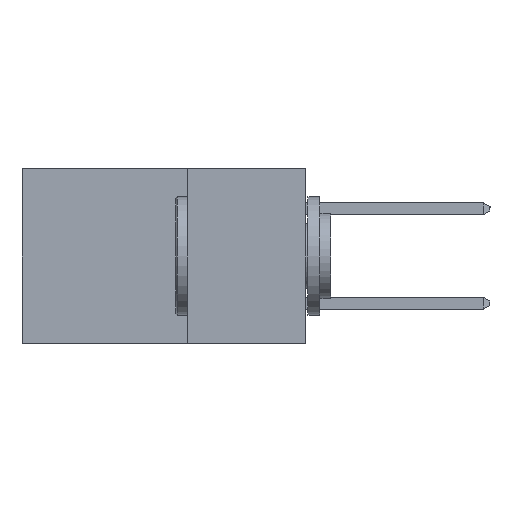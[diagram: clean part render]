
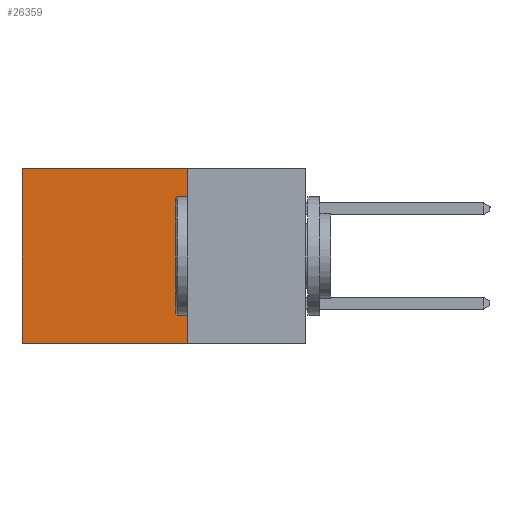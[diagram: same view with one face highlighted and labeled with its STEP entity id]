
A CAD part, left-side view. The second image highlights one B-rep face of the part: STEP entity #26359.
In plain terms, the highlighted planar face has unit normal (-1, 0, 0).
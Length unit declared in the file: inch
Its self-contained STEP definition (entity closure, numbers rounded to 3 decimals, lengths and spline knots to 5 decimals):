
#502 = CARTESIAN_POINT ( 'NONE',  ( 0.2615, 0.25, -0.37 ) ) ;
#1599 = EDGE_CURVE ( 'NONE', #26156, #15115, #1630, .T. ) ;
#1630 = LINE ( 'NONE', #23669, #22161 ) ;
#2135 = LINE ( 'NONE', #6465, #19818 ) ;
#2148 = LINE ( 'NONE', #24849, #10229 ) ;
#2182 = ORIENTED_EDGE ( 'NONE', *, *, #1599, .F. ) ;
#2357 = LINE ( 'NONE', #16408, #9030 ) ;
#4839 = PLANE ( 'NONE',  #10345 ) ;
#6465 = CARTESIAN_POINT ( 'NONE',  ( 0.2615, 0.6, -0.37 ) ) ;
#7989 = EDGE_CURVE ( 'NONE', #15115, #23376, #2148, .T. ) ;
#9030 = VECTOR ( 'NONE', #10595, 39.37008 ) ;
#9242 = VERTEX_POINT ( 'NONE', #22430 ) ;
#10229 = VECTOR ( 'NONE', #14302, 39.37008 ) ;
#10345 = AXIS2_PLACEMENT_3D ( 'NONE', #14966, #15353, #21310 ) ;
#10379 = CARTESIAN_POINT ( 'NONE',  ( 0.2615, 0.25, 0. ) ) ;
#10595 = DIRECTION ( 'NONE',  ( 0., 1., 0. ) ) ;
#12835 = EDGE_CURVE ( 'NONE', #9242, #23376, #2135, .T. ) ;
#13243 = EDGE_CURVE ( 'NONE', #26156, #9242, #2357, .T. ) ;
#13590 = CARTESIAN_POINT ( 'NONE',  ( 0.2615, 0.6, -0.37 ) ) ;
#14302 = DIRECTION ( 'NONE',  ( 0., 1., 0. ) ) ;
#14966 = CARTESIAN_POINT ( 'NONE',  ( 0.2615, 0.25, -0.37 ) ) ;
#15115 = VERTEX_POINT ( 'NONE', #502 ) ;
#15353 = DIRECTION ( 'NONE',  ( 1., 0., 0. ) ) ;
#16408 = CARTESIAN_POINT ( 'NONE',  ( 0.2615, 0.25, 0. ) ) ;
#16432 = ORIENTED_EDGE ( 'NONE', *, *, #12835, .T. ) ;
#19111 = ORIENTED_EDGE ( 'NONE', *, *, #13243, .T. ) ;
#19284 = FACE_OUTER_BOUND ( 'NONE', #21211, .T. ) ;
#19360 = ORIENTED_EDGE ( 'NONE', *, *, #7989, .F. ) ;
#19818 = VECTOR ( 'NONE', #22955, 39.37008 ) ;
#21211 = EDGE_LOOP ( 'NONE', ( #16432, #19360, #2182, #19111 ) ) ;
#21310 = DIRECTION ( 'NONE',  ( 0., 0., -1. ) ) ;
#21619 = DIRECTION ( 'NONE',  ( 0., 0., -1. ) ) ;
#22161 = VECTOR ( 'NONE', #21619, 39.37008 ) ;
#22430 = CARTESIAN_POINT ( 'NONE',  ( 0.2615, 0.6, 0. ) ) ;
#22955 = DIRECTION ( 'NONE',  ( 0., 0., -1. ) ) ;
#23376 = VERTEX_POINT ( 'NONE', #13590 ) ;
#23669 = CARTESIAN_POINT ( 'NONE',  ( 0.2615, 0.25, -0.37 ) ) ;
#24849 = CARTESIAN_POINT ( 'NONE',  ( 0.2615, 0.25, -0.37 ) ) ;
#26156 = VERTEX_POINT ( 'NONE', #10379 ) ;
#26359 = ADVANCED_FACE ( 'NONE', ( #19284 ), #4839, .F. ) ;
